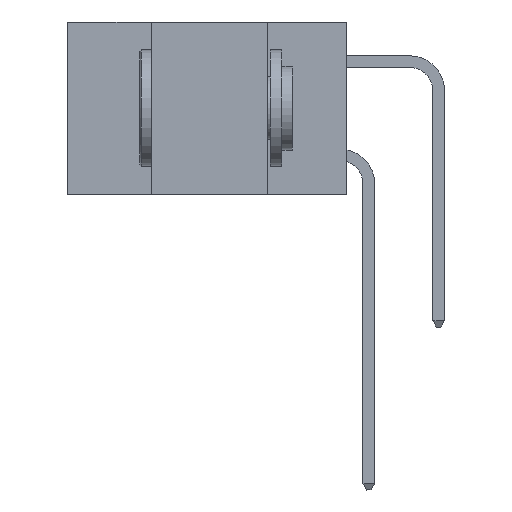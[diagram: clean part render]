
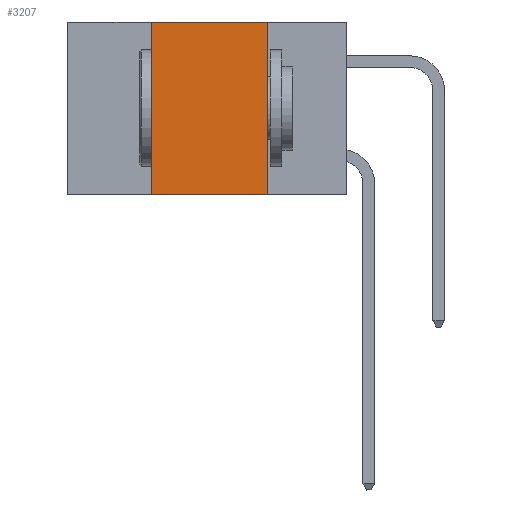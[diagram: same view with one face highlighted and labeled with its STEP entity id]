
A CAD part, left-side view. The second image highlights one B-rep face of the part: STEP entity #3207.
In plain terms, the highlighted planar face has unit normal (-1, 0, 0).
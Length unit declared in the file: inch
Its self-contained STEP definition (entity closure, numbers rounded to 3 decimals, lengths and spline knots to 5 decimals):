
#378 = DIRECTION ( 'NONE',  ( 0., 0., -1. ) ) ;
#2490 = CARTESIAN_POINT ( 'NONE',  ( 0., 0.6, 0. ) ) ;
#3207 = ADVANCED_FACE ( 'NONE', ( #16418 ), #15728, .F. ) ;
#4029 = LINE ( 'NONE', #25375, #24479 ) ;
#4073 = VECTOR ( 'NONE', #8153, 39.37008 ) ;
#4658 = EDGE_CURVE ( 'NONE', #6930, #4952, #4029, .T. ) ;
#4701 = CARTESIAN_POINT ( 'NONE',  ( 0., 0.42, 0. ) ) ;
#4952 = VERTEX_POINT ( 'NONE', #17652 ) ;
#5194 = EDGE_LOOP ( 'NONE', ( #5219, #28002, #5980, #24864 ) ) ;
#5219 = ORIENTED_EDGE ( 'NONE', *, *, #4658, .F. ) ;
#5393 = VERTEX_POINT ( 'NONE', #20798 ) ;
#5980 = ORIENTED_EDGE ( 'NONE', *, *, #26442, .F. ) ;
#6117 = DIRECTION ( 'NONE',  ( 0., -1., 0. ) ) ;
#6634 = AXIS2_PLACEMENT_3D ( 'NONE', #2490, #24305, #378 ) ;
#6930 = VERTEX_POINT ( 'NONE', #15824 ) ;
#8153 = DIRECTION ( 'NONE',  ( 0., -1., 0. ) ) ;
#9237 = EDGE_CURVE ( 'NONE', #5393, #4952, #22883, .T. ) ;
#11730 = LINE ( 'NONE', #4701, #18557 ) ;
#12025 = DIRECTION ( 'NONE',  ( 0., 0., -1. ) ) ;
#13594 = LINE ( 'NONE', #15001, #4073 ) ;
#14631 = VERTEX_POINT ( 'NONE', #26732 ) ;
#15001 = CARTESIAN_POINT ( 'NONE',  ( 0., 0.6, 0. ) ) ;
#15728 = PLANE ( 'NONE',  #6634 ) ;
#15824 = CARTESIAN_POINT ( 'NONE',  ( 0., 0.17, 0. ) ) ;
#16392 = CARTESIAN_POINT ( 'NONE',  ( 0., 0.6, -0.37 ) ) ;
#16418 = FACE_OUTER_BOUND ( 'NONE', #5194, .T. ) ;
#17652 = CARTESIAN_POINT ( 'NONE',  ( 0., 0.17, -0.37 ) ) ;
#18557 = VECTOR ( 'NONE', #26712, 39.37008 ) ;
#18711 = EDGE_CURVE ( 'NONE', #14631, #6930, #13594, .T. ) ;
#20798 = CARTESIAN_POINT ( 'NONE',  ( 0., 0.42, -0.37 ) ) ;
#22883 = LINE ( 'NONE', #16392, #25929 ) ;
#24305 = DIRECTION ( 'NONE',  ( 1., 0., 0. ) ) ;
#24479 = VECTOR ( 'NONE', #12025, 39.37008 ) ;
#24864 = ORIENTED_EDGE ( 'NONE', *, *, #9237, .T. ) ;
#25375 = CARTESIAN_POINT ( 'NONE',  ( 0., 0.17, 0. ) ) ;
#25929 = VECTOR ( 'NONE', #6117, 39.37008 ) ;
#26442 = EDGE_CURVE ( 'NONE', #5393, #14631, #11730, .T. ) ;
#26712 = DIRECTION ( 'NONE',  ( 0., 0., 1. ) ) ;
#26732 = CARTESIAN_POINT ( 'NONE',  ( 0., 0.42, 0. ) ) ;
#28002 = ORIENTED_EDGE ( 'NONE', *, *, #18711, .F. ) ;
